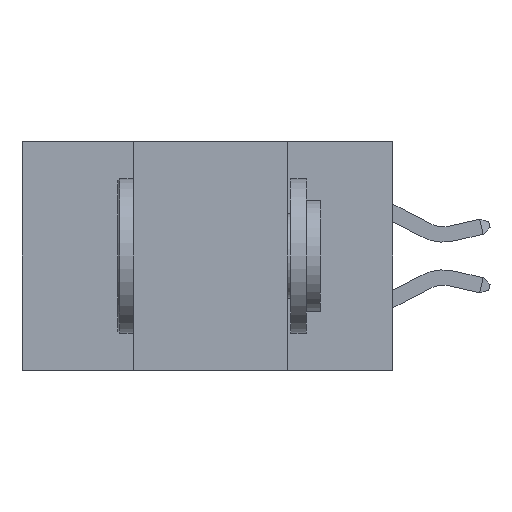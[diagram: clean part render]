
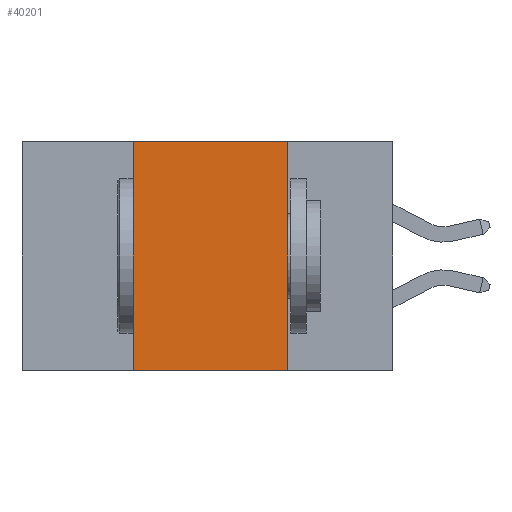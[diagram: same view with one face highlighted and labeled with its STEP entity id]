
A CAD part, left-side view. The second image highlights one B-rep face of the part: STEP entity #40201.
In plain terms, the highlighted planar face has unit normal (-1, 0, 0).
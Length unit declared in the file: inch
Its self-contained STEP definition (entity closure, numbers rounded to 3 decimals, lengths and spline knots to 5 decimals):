
#347 = EDGE_CURVE ( 'NONE', #2288, #32583, #14824, .T. ) ;
#1720 = ORIENTED_EDGE ( 'NONE', *, *, #21961, .T. ) ;
#2193 = LINE ( 'NONE', #41157, #36639 ) ;
#2216 = DIRECTION ( 'NONE',  ( 0., -1., 0. ) ) ;
#2288 = VERTEX_POINT ( 'NONE', #28752 ) ;
#3317 = VERTEX_POINT ( 'NONE', #14595 ) ;
#3375 = DIRECTION ( 'NONE',  ( 0., -1., 0. ) ) ;
#5886 = VECTOR ( 'NONE', #3375, 39.37008 ) ;
#6344 = EDGE_CURVE ( 'NONE', #3317, #2288, #2193, .T. ) ;
#7000 = CARTESIAN_POINT ( 'NONE',  ( 0., 0.6, 0. ) ) ;
#7636 = ORIENTED_EDGE ( 'NONE', *, *, #6344, .F. ) ;
#11004 = DIRECTION ( 'NONE',  ( 0., 0., -1. ) ) ;
#11472 = DIRECTION ( 'NONE',  ( 0., 0., 1. ) ) ;
#12336 = ORIENTED_EDGE ( 'NONE', *, *, #347, .F. ) ;
#14081 = CARTESIAN_POINT ( 'NONE',  ( 0., 0.17, 0. ) ) ;
#14216 = PLANE ( 'NONE',  #30683 ) ;
#14595 = CARTESIAN_POINT ( 'NONE',  ( 0., 0.42, -0.37 ) ) ;
#14824 = LINE ( 'NONE', #7000, #5886 ) ;
#15932 = FACE_OUTER_BOUND ( 'NONE', #18489, .T. ) ;
#18489 = EDGE_LOOP ( 'NONE', ( #26920, #12336, #7636, #1720 ) ) ;
#21131 = LINE ( 'NONE', #29010, #27826 ) ;
#21961 = EDGE_CURVE ( 'NONE', #3317, #28078, #21131, .T. ) ;
#23619 = CARTESIAN_POINT ( 'NONE',  ( 0., 0.17, 0. ) ) ;
#24269 = CARTESIAN_POINT ( 'NONE',  ( 0., 0.6, 0. ) ) ;
#26611 = CARTESIAN_POINT ( 'NONE',  ( 0., 0.17, -0.37 ) ) ;
#26920 = ORIENTED_EDGE ( 'NONE', *, *, #36703, .F. ) ;
#27826 = VECTOR ( 'NONE', #2216, 39.37008 ) ;
#28078 = VERTEX_POINT ( 'NONE', #26611 ) ;
#28752 = CARTESIAN_POINT ( 'NONE',  ( 0., 0.42, 0. ) ) ;
#29010 = CARTESIAN_POINT ( 'NONE',  ( 0., 0.6, -0.37 ) ) ;
#30235 = DIRECTION ( 'NONE',  ( 0., 0., -1. ) ) ;
#30683 = AXIS2_PLACEMENT_3D ( 'NONE', #24269, #30897, #11004 ) ;
#30897 = DIRECTION ( 'NONE',  ( 1., 0., 0. ) ) ;
#32583 = VERTEX_POINT ( 'NONE', #14081 ) ;
#32990 = LINE ( 'NONE', #23619, #40747 ) ;
#36639 = VECTOR ( 'NONE', #11472, 39.37008 ) ;
#36703 = EDGE_CURVE ( 'NONE', #32583, #28078, #32990, .T. ) ;
#40201 = ADVANCED_FACE ( 'NONE', ( #15932 ), #14216, .F. ) ;
#40747 = VECTOR ( 'NONE', #30235, 39.37008 ) ;
#41157 = CARTESIAN_POINT ( 'NONE',  ( 0., 0.42, 0. ) ) ;
